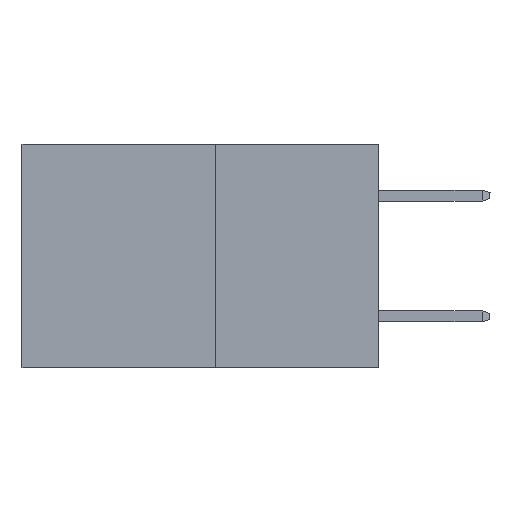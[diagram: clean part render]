
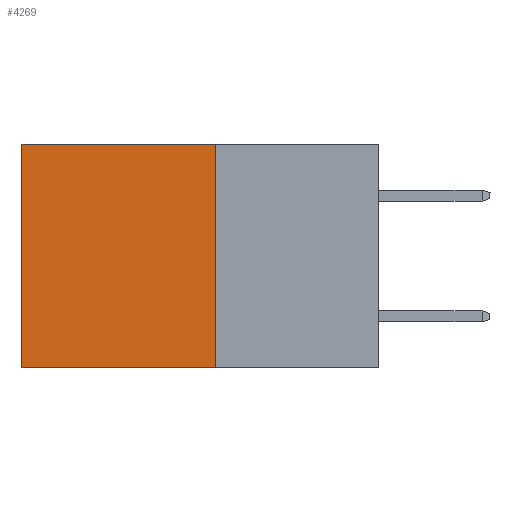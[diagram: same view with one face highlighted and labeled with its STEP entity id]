
A CAD part, left-side view. The second image highlights one B-rep face of the part: STEP entity #4269.
In plain terms, the highlighted planar face has unit normal (-1, 0, 0).
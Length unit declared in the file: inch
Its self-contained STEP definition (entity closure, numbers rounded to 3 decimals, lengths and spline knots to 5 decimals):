
#221 = ORIENTED_EDGE ( 'NONE', *, *, #7557, .F. ) ;
#370 = CARTESIAN_POINT ( 'NONE',  ( 0.277, 0.27, -0.37 ) ) ;
#660 = VERTEX_POINT ( 'NONE', #8649 ) ;
#1232 = DIRECTION ( 'NONE',  ( 0., 0., -1. ) ) ;
#2081 = VECTOR ( 'NONE', #9341, 39.37008 ) ;
#2374 = LINE ( 'NONE', #8507, #2081 ) ;
#2568 = ORIENTED_EDGE ( 'NONE', *, *, #4305, .T. ) ;
#2624 = VERTEX_POINT ( 'NONE', #4544 ) ;
#3053 = AXIS2_PLACEMENT_3D ( 'NONE', #8179, #8009, #7685 ) ;
#3357 = EDGE_LOOP ( 'NONE', ( #2568, #9619, #221, #5399 ) ) ;
#4088 = CARTESIAN_POINT ( 'NONE',  ( 0.277, 0.27, -0.37 ) ) ;
#4269 = ADVANCED_FACE ( 'NONE', ( #10475 ), #8167, .F. ) ;
#4305 = EDGE_CURVE ( 'NONE', #9906, #660, #5994, .T. ) ;
#4544 = CARTESIAN_POINT ( 'NONE',  ( 0.277, 0.27, 0. ) ) ;
#5399 = ORIENTED_EDGE ( 'NONE', *, *, #5751, .T. ) ;
#5521 = VERTEX_POINT ( 'NONE', #370 ) ;
#5627 = LINE ( 'NONE', #10200, #9829 ) ;
#5751 = EDGE_CURVE ( 'NONE', #2624, #9906, #5627, .T. ) ;
#5994 = LINE ( 'NONE', #7202, #10201 ) ;
#6890 = DIRECTION ( 'NONE',  ( 0., 0., -1. ) ) ;
#7202 = CARTESIAN_POINT ( 'NONE',  ( 0.277, 0.59, -0.37 ) ) ;
#7557 = EDGE_CURVE ( 'NONE', #2624, #5521, #11396, .T. ) ;
#7685 = DIRECTION ( 'NONE',  ( 0., 0., -1. ) ) ;
#8009 = DIRECTION ( 'NONE',  ( 1., 0., 0. ) ) ;
#8167 = PLANE ( 'NONE',  #3053 ) ;
#8179 = CARTESIAN_POINT ( 'NONE',  ( 0.277, 0.27, -0.37 ) ) ;
#8448 = CARTESIAN_POINT ( 'NONE',  ( 0.277, 0.59, 0. ) ) ;
#8507 = CARTESIAN_POINT ( 'NONE',  ( 0.277, 0.27, -0.37 ) ) ;
#8649 = CARTESIAN_POINT ( 'NONE',  ( 0.277, 0.59, -0.37 ) ) ;
#9116 = VECTOR ( 'NONE', #1232, 39.37008 ) ;
#9319 = DIRECTION ( 'NONE',  ( 0., 1., 0. ) ) ;
#9341 = DIRECTION ( 'NONE',  ( 0., 1., 0. ) ) ;
#9619 = ORIENTED_EDGE ( 'NONE', *, *, #10751, .F. ) ;
#9829 = VECTOR ( 'NONE', #9319, 39.37008 ) ;
#9906 = VERTEX_POINT ( 'NONE', #8448 ) ;
#10200 = CARTESIAN_POINT ( 'NONE',  ( 0.277, 0.27, 0. ) ) ;
#10201 = VECTOR ( 'NONE', #6890, 39.37008 ) ;
#10475 = FACE_OUTER_BOUND ( 'NONE', #3357, .T. ) ;
#10751 = EDGE_CURVE ( 'NONE', #5521, #660, #2374, .T. ) ;
#11396 = LINE ( 'NONE', #4088, #9116 ) ;
